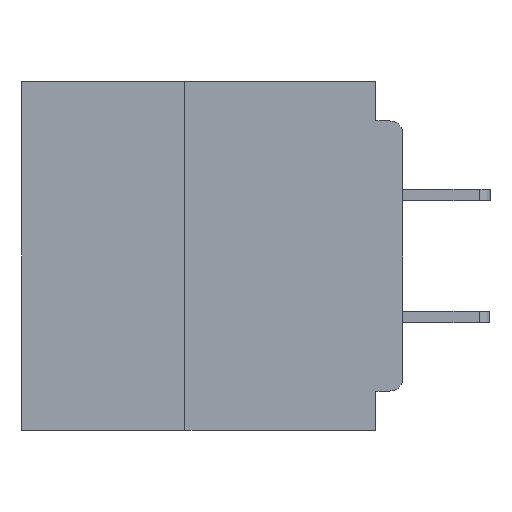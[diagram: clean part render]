
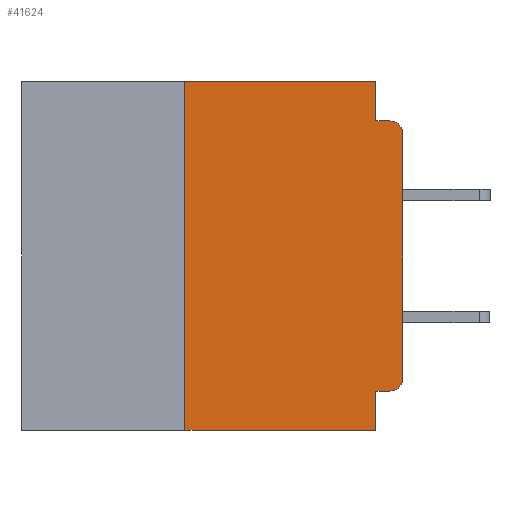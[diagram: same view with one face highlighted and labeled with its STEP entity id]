
A CAD part, left-side view. The second image highlights one B-rep face of the part: STEP entity #41624.
In plain terms, the highlighted planar face has unit normal (-1, 0, 0).
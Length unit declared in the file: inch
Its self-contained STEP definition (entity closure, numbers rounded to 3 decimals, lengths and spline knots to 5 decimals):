
#162 = ORIENTED_EDGE ( 'NONE', *, *, #14143, .T. ) ;
#440 = VERTEX_POINT ( 'NONE', #18851 ) ;
#1169 = CARTESIAN_POINT ( 'NONE',  ( 0., 0.031, -0.045 ) ) ;
#1200 = VERTEX_POINT ( 'NONE', #42740 ) ;
#1296 = ORIENTED_EDGE ( 'NONE', *, *, #14629, .F. ) ;
#2520 = CIRCLE ( 'NONE', #42449, 0.015 ) ;
#2575 = DIRECTION ( 'NONE',  ( 1., 0., 0. ) ) ;
#3290 = DIRECTION ( 'NONE',  ( 0., 0., 1. ) ) ;
#3334 = CARTESIAN_POINT ( 'NONE',  ( 0., 0.031, 0. ) ) ;
#3475 = LINE ( 'NONE', #50630, #46138 ) ;
#4752 = ORIENTED_EDGE ( 'NONE', *, *, #6504, .T. ) ;
#5412 = VECTOR ( 'NONE', #32960, 39.37008 ) ;
#5413 = ORIENTED_EDGE ( 'NONE', *, *, #8240, .F. ) ;
#5527 = EDGE_CURVE ( 'NONE', #20986, #7168, #40323, .T. ) ;
#6504 = EDGE_CURVE ( 'NONE', #1200, #21917, #3475, .T. ) ;
#7146 = LINE ( 'NONE', #29064, #39799 ) ;
#7168 = VERTEX_POINT ( 'NONE', #21140 ) ;
#7785 = DIRECTION ( 'NONE',  ( 0., -1., 0. ) ) ;
#8240 = EDGE_CURVE ( 'NONE', #440, #19989, #53297, .T. ) ;
#9458 = AXIS2_PLACEMENT_3D ( 'NONE', #23606, #53213, #27900 ) ;
#10156 = VERTEX_POINT ( 'NONE', #13273 ) ;
#10507 = CARTESIAN_POINT ( 'NONE',  ( 0., 0.25, 0. ) ) ;
#10691 = EDGE_CURVE ( 'NONE', #29026, #10156, #7146, .T. ) ;
#13273 = CARTESIAN_POINT ( 'NONE',  ( 0., 0.031, -0.4 ) ) ;
#13981 = CARTESIAN_POINT ( 'NONE',  ( 0., 0., -0.045 ) ) ;
#14143 = EDGE_CURVE ( 'NONE', #440, #1200, #30131, .T. ) ;
#14222 = CARTESIAN_POINT ( 'NONE',  ( 0., 0.25, -0.4 ) ) ;
#14629 = EDGE_CURVE ( 'NONE', #54400, #52142, #28722, .T. ) ;
#15116 = AXIS2_PLACEMENT_3D ( 'NONE', #28224, #2575, #32515 ) ;
#15544 = ORIENTED_EDGE ( 'NONE', *, *, #44863, .T. ) ;
#15920 = CARTESIAN_POINT ( 'NONE',  ( 0., 0.031, -0.355 ) ) ;
#16674 = EDGE_CURVE ( 'NONE', #29026, #54400, #33823, .T. ) ;
#16689 = DIRECTION ( 'NONE',  ( 0., 0., 1. ) ) ;
#17929 = EDGE_LOOP ( 'NONE', ( #4752, #15544, #23214, #46776, #1296, #41747, #19292, #42872, #5413, #162 ) ) ;
#18851 = CARTESIAN_POINT ( 'NONE',  ( 0., 0.015, -0.355 ) ) ;
#18937 = FACE_OUTER_BOUND ( 'NONE', #17929, .T. ) ;
#19292 = ORIENTED_EDGE ( 'NONE', *, *, #10691, .T. ) ;
#19667 = PLANE ( 'NONE',  #15116 ) ;
#19989 = VERTEX_POINT ( 'NONE', #15920 ) ;
#20986 = VERTEX_POINT ( 'NONE', #1169 ) ;
#21140 = CARTESIAN_POINT ( 'NONE',  ( 0., 0.015, -0.045 ) ) ;
#21917 = VERTEX_POINT ( 'NONE', #45178 ) ;
#23173 = DIRECTION ( 'NONE',  ( -1., 0., 0. ) ) ;
#23214 = ORIENTED_EDGE ( 'NONE', *, *, #5527, .F. ) ;
#23606 = CARTESIAN_POINT ( 'NONE',  ( 0., 0.015, -0.34 ) ) ;
#27705 = DIRECTION ( 'NONE',  ( 0., 0., -1. ) ) ;
#27900 = DIRECTION ( 'NONE',  ( 0., 0., -1. ) ) ;
#28224 = CARTESIAN_POINT ( 'NONE',  ( 0., 0.437, 0. ) ) ;
#28416 = CARTESIAN_POINT ( 'NONE',  ( 0., 0.031, -0.4 ) ) ;
#28722 = LINE ( 'NONE', #40089, #38673 ) ;
#29026 = VERTEX_POINT ( 'NONE', #14222 ) ;
#29064 = CARTESIAN_POINT ( 'NONE',  ( 0., 0.437, -0.4 ) ) ;
#30131 = CIRCLE ( 'NONE', #9458, 0.015 ) ;
#30567 = VECTOR ( 'NONE', #53736, 39.37008 ) ;
#32515 = DIRECTION ( 'NONE',  ( 0., 0., -1. ) ) ;
#32960 = DIRECTION ( 'NONE',  ( 0., 1., 0. ) ) ;
#33823 = LINE ( 'NONE', #54247, #54916 ) ;
#34419 = LINE ( 'NONE', #40305, #54223 ) ;
#37925 = EDGE_CURVE ( 'NONE', #52142, #20986, #34419, .T. ) ;
#38673 = VECTOR ( 'NONE', #52820, 39.37008 ) ;
#38991 = VECTOR ( 'NONE', #47924, 39.37008 ) ;
#39799 = VECTOR ( 'NONE', #7785, 39.37008 ) ;
#40089 = CARTESIAN_POINT ( 'NONE',  ( 0., 0.437, 0. ) ) ;
#40305 = CARTESIAN_POINT ( 'NONE',  ( 0., 0.031, 0. ) ) ;
#40323 = LINE ( 'NONE', #13981, #38991 ) ;
#41624 = ADVANCED_FACE ( 'NONE', ( #18937 ), #19667, .F. ) ;
#41747 = ORIENTED_EDGE ( 'NONE', *, *, #16674, .F. ) ;
#41784 = LINE ( 'NONE', #28416, #30567 ) ;
#42449 = AXIS2_PLACEMENT_3D ( 'NONE', #48575, #23173, #52814 ) ;
#42740 = CARTESIAN_POINT ( 'NONE',  ( 0., 0., -0.34 ) ) ;
#42872 = ORIENTED_EDGE ( 'NONE', *, *, #49243, .F. ) ;
#44863 = EDGE_CURVE ( 'NONE', #21917, #7168, #2520, .T. ) ;
#45178 = CARTESIAN_POINT ( 'NONE',  ( 0., 0., -0.06 ) ) ;
#46138 = VECTOR ( 'NONE', #16689, 39.37008 ) ;
#46776 = ORIENTED_EDGE ( 'NONE', *, *, #37925, .F. ) ;
#47924 = DIRECTION ( 'NONE',  ( 0., -1., 0. ) ) ;
#48575 = CARTESIAN_POINT ( 'NONE',  ( 0., 0.015, -0.06 ) ) ;
#49243 = EDGE_CURVE ( 'NONE', #19989, #10156, #41784, .T. ) ;
#50630 = CARTESIAN_POINT ( 'NONE',  ( 0., 0., 0. ) ) ;
#52142 = VERTEX_POINT ( 'NONE', #3334 ) ;
#52814 = DIRECTION ( 'NONE',  ( 0., 0., -1. ) ) ;
#52820 = DIRECTION ( 'NONE',  ( 0., -1., 0. ) ) ;
#53213 = DIRECTION ( 'NONE',  ( -1., 0., 0. ) ) ;
#53297 = LINE ( 'NONE', #53993, #5412 ) ;
#53736 = DIRECTION ( 'NONE',  ( 0., 0., -1. ) ) ;
#53993 = CARTESIAN_POINT ( 'NONE',  ( 0., 0., -0.355 ) ) ;
#54223 = VECTOR ( 'NONE', #27705, 39.37008 ) ;
#54247 = CARTESIAN_POINT ( 'NONE',  ( 0., 0.25, -0.4 ) ) ;
#54400 = VERTEX_POINT ( 'NONE', #10507 ) ;
#54916 = VECTOR ( 'NONE', #3290, 39.37008 ) ;
